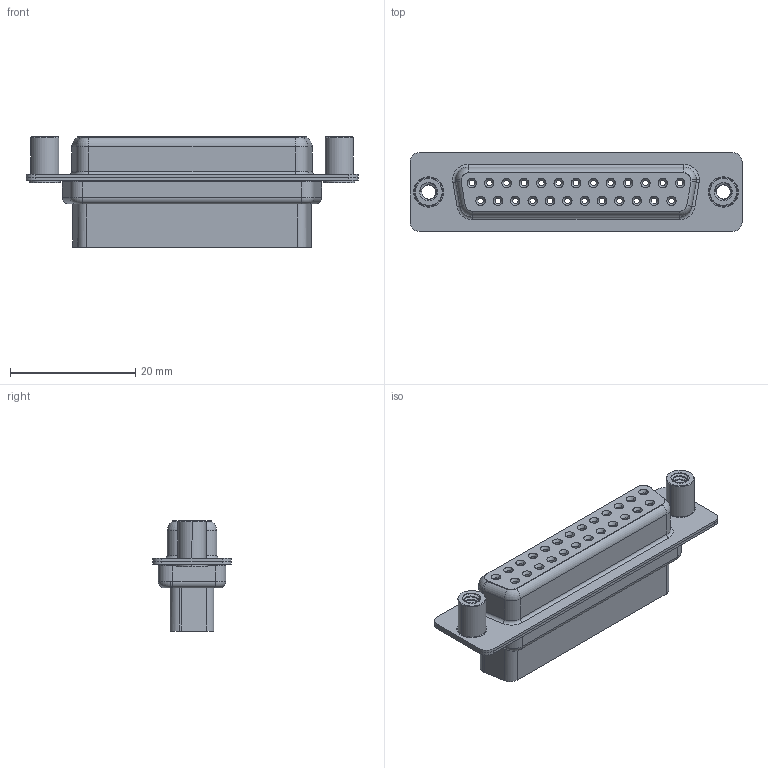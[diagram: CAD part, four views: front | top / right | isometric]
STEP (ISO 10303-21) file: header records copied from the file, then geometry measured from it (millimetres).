
FILE_DESCRIPTION (( 'STEP AP203' ), '1' );
FILE_NAME ('628-025-010-048.STEP', '2020-07-15T20:29:50', ( '' ), ( '' ), 'SwSTEP 2.0', 'SolidWorks 2020', '' );
FILE_SCHEMA (( 'CONFIG_CONTROL_DESIGN' ));
Length unit declared in the file: millimetre
Products named in the file (5): 628 Housing_25 HP; 628 4-40 Threaded Standoff; 628 Shell Rear_25 Contacts; 628 Shell Front_25 Contacts; 628-025-010-048
Assembly tree (5 placements, depth 2):
  628-025-010-048
    628 Housing_25 HP
    628 Shell Front_25 Contacts
    628 Shell Rear_25 Contacts
    628 4-40 Threaded Standoff  x2
Bounding box: 53 x 12.6 x 17.6 mm (x, y, z)
Volume: 4741.5 mm3; surface area: 8163.5 mm2
Topology: 5 solids, 5 shells, 638 faces, 1479 edges, 939 vertices
Faces by surface type: cylinder 365, plane 144, torus 63, cone 60, bspline 6
Entity records: 19192 total; most frequent: CARTESIAN_POINT 4775, DIRECTION 3171, ORIENTED_EDGE 2702, EDGE_CURVE 1351, AXIS2_PLACEMENT_3D 1330, VERTEX_POINT 856, CIRCLE 737, EDGE_LOOP 737
